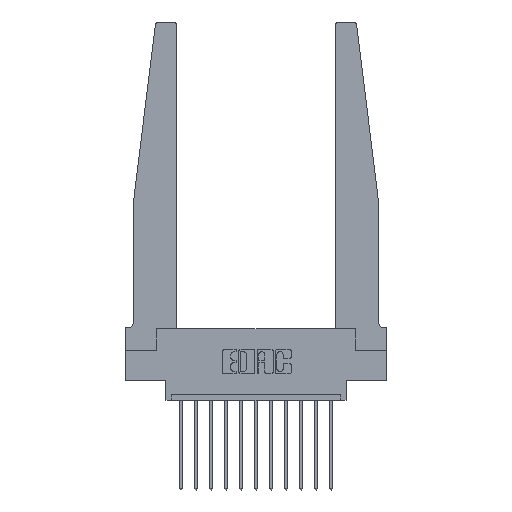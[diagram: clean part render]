
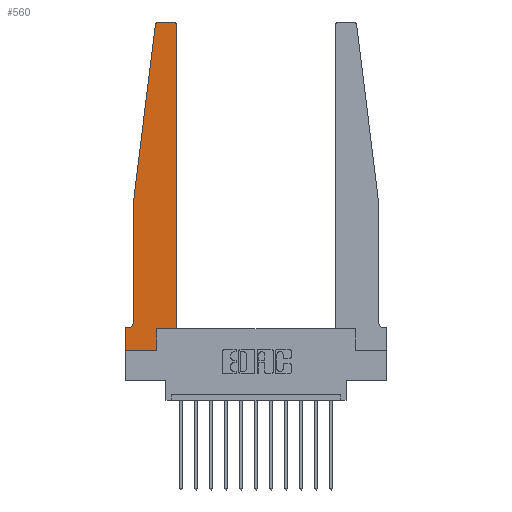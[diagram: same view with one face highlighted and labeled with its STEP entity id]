
A CAD part, top view. The second image highlights one B-rep face of the part: STEP entity #560.
In plain terms, the highlighted planar face has unit normal (0, 0, 1).
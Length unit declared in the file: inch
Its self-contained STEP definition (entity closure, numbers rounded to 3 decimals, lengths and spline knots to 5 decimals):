
#100 = VECTOR ( 'NONE', #4839, 39.37008 ) ;
#441 = ORIENTED_EDGE ( 'NONE', *, *, #1985, .T. ) ;
#530 = LINE ( 'NONE', #4319, #2609 ) ;
#560 = ADVANCED_FACE ( 'NONE', ( #1596 ), #10950, .T. ) ;
#743 = CARTESIAN_POINT ( 'NONE',  ( 0.425, 0.18, 0.37 ) ) ;
#954 = CARTESIAN_POINT ( 'NONE',  ( 0.27653, 2.72, 0.37 ) ) ;
#1596 = FACE_OUTER_BOUND ( 'NONE', #7153, .T. ) ;
#1634 = EDGE_CURVE ( 'NONE', #3386, #11347, #1737, .T. ) ;
#1735 = CARTESIAN_POINT ( 'NONE',  ( 0., 0., 0.37 ) ) ;
#1737 = CIRCLE ( 'NONE', #8845, 0.03 ) ;
#1751 = CARTESIAN_POINT ( 'NONE',  ( 0.425, 2.72, 0.37 ) ) ;
#1786 = DIRECTION ( 'NONE',  ( 1., 0., 0. ) ) ;
#1985 = EDGE_CURVE ( 'NONE', #6457, #11861, #14911, .T. ) ;
#2075 = DIRECTION ( 'NONE',  ( 1., 0., 0. ) ) ;
#2247 = VERTEX_POINT ( 'NONE', #7097 ) ;
#2609 = VECTOR ( 'NONE', #10603, 39.37008 ) ;
#2680 = CARTESIAN_POINT ( 'NONE',  ( 0.395, 2.75, 0.37 ) ) ;
#3386 = VERTEX_POINT ( 'NONE', #4455 ) ;
#3529 = VECTOR ( 'NONE', #3958, 39.37008 ) ;
#3694 = CARTESIAN_POINT ( 'NONE',  ( 0., 0., 0.37 ) ) ;
#3793 = CARTESIAN_POINT ( 'NONE',  ( 0.2605, 0.18, 0.37 ) ) ;
#3901 = LINE ( 'NONE', #11024, #100 ) ;
#3958 = DIRECTION ( 'NONE',  ( 0., -1., 0. ) ) ;
#4068 = EDGE_CURVE ( 'NONE', #11861, #12960, #12165, .T. ) ;
#4115 = CARTESIAN_POINT ( 'NONE',  ( 0.015, 0.1875, 0.37 ) ) ;
#4319 = CARTESIAN_POINT ( 'NONE',  ( 0., 0., 0.37 ) ) ;
#4394 = CARTESIAN_POINT ( 'NONE',  ( 0.015, 0.2375, 0.37 ) ) ;
#4455 = CARTESIAN_POINT ( 'NONE',  ( 0.27653, 2.75, 0.37 ) ) ;
#4479 = ORIENTED_EDGE ( 'NONE', *, *, #9426, .T. ) ;
#4604 = CARTESIAN_POINT ( 'NONE',  ( 0.065, 1.25, 0.37 ) ) ;
#4638 = VECTOR ( 'NONE', #10652, 39.37008 ) ;
#4639 = LINE ( 'NONE', #3694, #3529 ) ;
#4714 = DIRECTION ( 'NONE',  ( 0., 0., 1. ) ) ;
#4728 = ORIENTED_EDGE ( 'NONE', *, *, #8692, .T. ) ;
#4839 = DIRECTION ( 'NONE',  ( -1., 0., 0. ) ) ;
#5656 = DIRECTION ( 'NONE',  ( 0., 0., 1. ) ) ;
#5773 = DIRECTION ( 'NONE',  ( -1., 0., 0. ) ) ;
#5990 = CARTESIAN_POINT ( 'NONE',  ( 0.2605, 0.18, 0.37 ) ) ;
#5997 = DIRECTION ( 'NONE',  ( 1., 0., 0. ) ) ;
#6095 = AXIS2_PLACEMENT_3D ( 'NONE', #10790, #4714, #5997 ) ;
#6133 = ORIENTED_EDGE ( 'NONE', *, *, #12160, .T. ) ;
#6258 = ORIENTED_EDGE ( 'NONE', *, *, #15691, .T. ) ;
#6360 = CARTESIAN_POINT ( 'NONE',  ( 0.2605, 0., 0.37 ) ) ;
#6396 = EDGE_CURVE ( 'NONE', #2247, #11377, #15023, .T. ) ;
#6457 = VERTEX_POINT ( 'NONE', #5990 ) ;
#6519 = EDGE_CURVE ( 'NONE', #11347, #10986, #11545, .T. ) ;
#6553 = CARTESIAN_POINT ( 'NONE',  ( 0.425, 0.18, 0.37 ) ) ;
#6621 = ORIENTED_EDGE ( 'NONE', *, *, #1634, .T. ) ;
#7097 = CARTESIAN_POINT ( 'NONE',  ( 0.065, 0.2375, 0.37 ) ) ;
#7153 = EDGE_LOOP ( 'NONE', ( #9821, #6621, #14244, #4728, #9077, #6258, #13176, #8616, #6133, #441, #9860, #4479 ) ) ;
#7460 = CARTESIAN_POINT ( 'NONE',  ( 0.395, 2.72, 0.37 ) ) ;
#8181 = VERTEX_POINT ( 'NONE', #12731 ) ;
#8225 = VECTOR ( 'NONE', #13284, 39.37008 ) ;
#8320 = VECTOR ( 'NONE', #1786, 39.37008 ) ;
#8616 = ORIENTED_EDGE ( 'NONE', *, *, #9361, .T. ) ;
#8639 = DIRECTION ( 'NONE',  ( 0., 0., 1. ) ) ;
#8692 = EDGE_CURVE ( 'NONE', #10986, #2247, #12688, .T. ) ;
#8845 = AXIS2_PLACEMENT_3D ( 'NONE', #954, #5656, #2075 ) ;
#9059 = CARTESIAN_POINT ( 'NONE',  ( 0.065, 1.25, 0.37 ) ) ;
#9077 = ORIENTED_EDGE ( 'NONE', *, *, #6396, .T. ) ;
#9361 = EDGE_CURVE ( 'NONE', #12434, #11272, #530, .T. ) ;
#9426 = EDGE_CURVE ( 'NONE', #12960, #13233, #10887, .T. ) ;
#9821 = ORIENTED_EDGE ( 'NONE', *, *, #11027, .T. ) ;
#9827 = AXIS2_PLACEMENT_3D ( 'NONE', #7460, #8639, #10018 ) ;
#9828 = AXIS2_PLACEMENT_3D ( 'NONE', #4394, #11933, #5773 ) ;
#9860 = ORIENTED_EDGE ( 'NONE', *, *, #4068, .T. ) ;
#10018 = DIRECTION ( 'NONE',  ( 1., 0., 0. ) ) ;
#10426 = VECTOR ( 'NONE', #11663, 39.37008 ) ;
#10526 = DIRECTION ( 'NONE',  ( 0., -1., 0. ) ) ;
#10603 = DIRECTION ( 'NONE',  ( 1., 0., 0. ) ) ;
#10652 = DIRECTION ( 'NONE',  ( -1., 0., 0. ) ) ;
#10790 = CARTESIAN_POINT ( 'NONE',  ( 0., 0.1875, 0.37 ) ) ;
#10817 = VECTOR ( 'NONE', #14914, 39.37008 ) ;
#10887 = CIRCLE ( 'NONE', #9827, 0.03 ) ;
#10950 = PLANE ( 'NONE',  #6095 ) ;
#10986 = VERTEX_POINT ( 'NONE', #11894 ) ;
#11024 = CARTESIAN_POINT ( 'NONE',  ( 0.065, 0.1875, 0.37 ) ) ;
#11027 = EDGE_CURVE ( 'NONE', #13233, #3386, #14537, .T. ) ;
#11272 = VERTEX_POINT ( 'NONE', #6360 ) ;
#11347 = VERTEX_POINT ( 'NONE', #12799 ) ;
#11377 = VERTEX_POINT ( 'NONE', #4115 ) ;
#11545 = LINE ( 'NONE', #4604, #8225 ) ;
#11663 = DIRECTION ( 'NONE',  ( 0., 1., 0. ) ) ;
#11861 = VERTEX_POINT ( 'NONE', #6553 ) ;
#11894 = CARTESIAN_POINT ( 'NONE',  ( 0.065, 1.25, 0.37 ) ) ;
#11933 = DIRECTION ( 'NONE',  ( 0., 0., -1. ) ) ;
#12099 = VECTOR ( 'NONE', #10526, 39.37008 ) ;
#12160 = EDGE_CURVE ( 'NONE', #11272, #6457, #14116, .T. ) ;
#12165 = LINE ( 'NONE', #743, #10426 ) ;
#12434 = VERTEX_POINT ( 'NONE', #1735 ) ;
#12619 = CARTESIAN_POINT ( 'NONE',  ( 0.425, 0.18, 0.37 ) ) ;
#12688 = LINE ( 'NONE', #9059, #12099 ) ;
#12731 = CARTESIAN_POINT ( 'NONE',  ( 0., 0.1875, 0.37 ) ) ;
#12799 = CARTESIAN_POINT ( 'NONE',  ( 0.24675, 2.72367, 0.37 ) ) ;
#12960 = VERTEX_POINT ( 'NONE', #1751 ) ;
#13176 = ORIENTED_EDGE ( 'NONE', *, *, #15623, .T. ) ;
#13233 = VERTEX_POINT ( 'NONE', #2680 ) ;
#13284 = DIRECTION ( 'NONE',  ( -0.122, -0.992, 0. ) ) ;
#13296 = CARTESIAN_POINT ( 'NONE',  ( 0.25, 2.75, 0.37 ) ) ;
#14116 = LINE ( 'NONE', #3793, #10817 ) ;
#14244 = ORIENTED_EDGE ( 'NONE', *, *, #6519, .T. ) ;
#14537 = LINE ( 'NONE', #13296, #4638 ) ;
#14911 = LINE ( 'NONE', #12619, #8320 ) ;
#14914 = DIRECTION ( 'NONE',  ( 0., 1., 0. ) ) ;
#15023 = CIRCLE ( 'NONE', #9828, 0.05 ) ;
#15623 = EDGE_CURVE ( 'NONE', #8181, #12434, #4639, .T. ) ;
#15691 = EDGE_CURVE ( 'NONE', #11377, #8181, #3901, .T. ) ;
